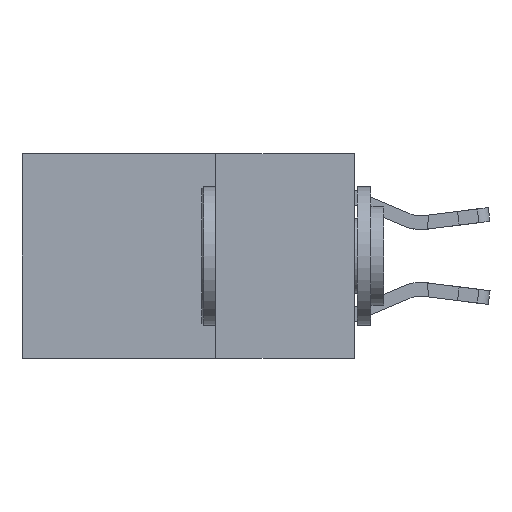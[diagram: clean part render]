
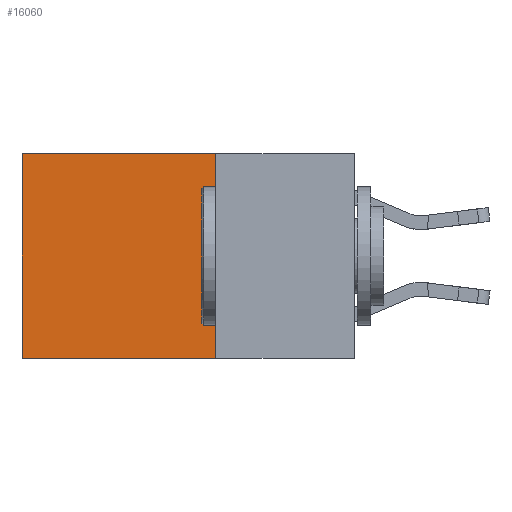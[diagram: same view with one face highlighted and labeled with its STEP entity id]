
A CAD part, left-side view. The second image highlights one B-rep face of the part: STEP entity #16060.
In plain terms, the highlighted planar face has unit normal (-1, 0, 0).
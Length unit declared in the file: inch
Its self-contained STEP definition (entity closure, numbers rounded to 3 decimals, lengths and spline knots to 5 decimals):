
#1698 = LINE ( 'NONE', #4538, #16888 ) ;
#2053 = CARTESIAN_POINT ( 'NONE',  ( 0.2625, 0.6, 0. ) ) ;
#2344 = CARTESIAN_POINT ( 'NONE',  ( 0.2625, 0.25, 0. ) ) ;
#2876 = VECTOR ( 'NONE', #16408, 39.37008 ) ;
#2969 = LINE ( 'NONE', #2053, #9857 ) ;
#3753 = CARTESIAN_POINT ( 'NONE',  ( 0.2625, 0.6, 0. ) ) ;
#4538 = CARTESIAN_POINT ( 'NONE',  ( 0.2625, 0.25, 0. ) ) ;
#4724 = VECTOR ( 'NONE', #9871, 39.37008 ) ;
#6250 = ORIENTED_EDGE ( 'NONE', *, *, #17840, .T. ) ;
#6928 = CARTESIAN_POINT ( 'NONE',  ( 0.2625, 0.25, -0.37 ) ) ;
#7286 = EDGE_CURVE ( 'NONE', #10639, #16578, #1698, .T. ) ;
#8106 = ORIENTED_EDGE ( 'NONE', *, *, #8426, .F. ) ;
#8271 = PLANE ( 'NONE',  #11724 ) ;
#8426 = EDGE_CURVE ( 'NONE', #16578, #11663, #18946, .T. ) ;
#8766 = CARTESIAN_POINT ( 'NONE',  ( 0.2625, 0.25, 0. ) ) ;
#9287 = EDGE_LOOP ( 'NONE', ( #11743, #8106, #17829, #6250 ) ) ;
#9783 = DIRECTION ( 'NONE',  ( 0., 0., -1. ) ) ;
#9857 = VECTOR ( 'NONE', #15920, 39.37008 ) ;
#9871 = DIRECTION ( 'NONE',  ( 0., 1., 0. ) ) ;
#10552 = EDGE_CURVE ( 'NONE', #16087, #11663, #2969, .T. ) ;
#10639 = VERTEX_POINT ( 'NONE', #8766 ) ;
#11663 = VERTEX_POINT ( 'NONE', #13083 ) ;
#11724 = AXIS2_PLACEMENT_3D ( 'NONE', #2344, #12909, #9783 ) ;
#11743 = ORIENTED_EDGE ( 'NONE', *, *, #10552, .T. ) ;
#12909 = DIRECTION ( 'NONE',  ( 1., 0., 0. ) ) ;
#13083 = CARTESIAN_POINT ( 'NONE',  ( 0.2625, 0.6, -0.37 ) ) ;
#13355 = CARTESIAN_POINT ( 'NONE',  ( 0.2625, 0.25, -0.37 ) ) ;
#13438 = CARTESIAN_POINT ( 'NONE',  ( 0.2625, 0.25, 0. ) ) ;
#14746 = LINE ( 'NONE', #13438, #2876 ) ;
#15920 = DIRECTION ( 'NONE',  ( 0., 0., -1. ) ) ;
#16060 = ADVANCED_FACE ( 'NONE', ( #16559 ), #8271, .F. ) ;
#16087 = VERTEX_POINT ( 'NONE', #3753 ) ;
#16408 = DIRECTION ( 'NONE',  ( 0., 1., 0. ) ) ;
#16559 = FACE_OUTER_BOUND ( 'NONE', #9287, .T. ) ;
#16578 = VERTEX_POINT ( 'NONE', #13355 ) ;
#16888 = VECTOR ( 'NONE', #18100, 39.37008 ) ;
#17829 = ORIENTED_EDGE ( 'NONE', *, *, #7286, .F. ) ;
#17840 = EDGE_CURVE ( 'NONE', #10639, #16087, #14746, .T. ) ;
#18100 = DIRECTION ( 'NONE',  ( 0., 0., -1. ) ) ;
#18946 = LINE ( 'NONE', #6928, #4724 ) ;
